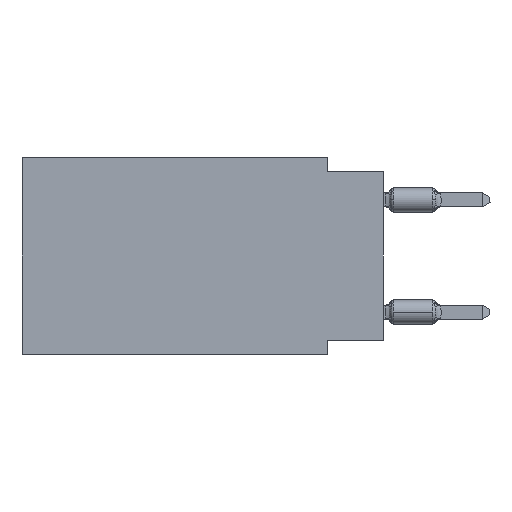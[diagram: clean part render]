
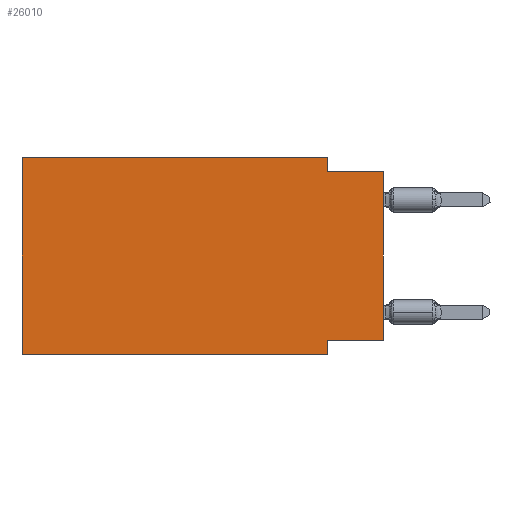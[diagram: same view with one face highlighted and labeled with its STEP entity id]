
A CAD part, left-side view. The second image highlights one B-rep face of the part: STEP entity #26010.
In plain terms, the highlighted planar face has unit normal (-1, 0, 0).
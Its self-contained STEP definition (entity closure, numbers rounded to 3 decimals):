
#1042 = PLANE ( 'NONE',  #23103 ) ;
#2280 = VECTOR ( 'NONE', #2632, 1000. ) ;
#2555 = VERTEX_POINT ( 'NONE', #8932 ) ;
#2632 = DIRECTION ( 'NONE',  ( 0., 1., 0. ) ) ;
#3701 = FACE_OUTER_BOUND ( 'NONE', #25335, .T. ) ;
#4126 = LINE ( 'NONE', #26616, #11478 ) ;
#4437 = LINE ( 'NONE', #19171, #16030 ) ;
#4621 = DIRECTION ( 'NONE',  ( 0., 0., -1. ) ) ;
#4666 = ORIENTED_EDGE ( 'NONE', *, *, #35360, .F. ) ;
#5027 = ORIENTED_EDGE ( 'NONE', *, *, #19436, .F. ) ;
#6119 = CARTESIAN_POINT ( 'NONE',  ( 0., 0., -0.635 ) ) ;
#6375 = DIRECTION ( 'NONE',  ( 0., 0., -1. ) ) ;
#6600 = DIRECTION ( 'NONE',  ( 0., 0., 1. ) ) ;
#7098 = LINE ( 'NONE', #16158, #21920 ) ;
#8932 = CARTESIAN_POINT ( 'NONE',  ( 0., 0., -0.635 ) ) ;
#9439 = VERTEX_POINT ( 'NONE', #15293 ) ;
#10919 = ORIENTED_EDGE ( 'NONE', *, *, #26098, .F. ) ;
#11478 = VECTOR ( 'NONE', #6600, 1000. ) ;
#12414 = DIRECTION ( 'NONE',  ( 1., 0., 0. ) ) ;
#12764 = DIRECTION ( 'NONE',  ( 0., -1., 0. ) ) ;
#13565 = CARTESIAN_POINT ( 'NONE',  ( 0., 2.54, -0.635 ) ) ;
#14224 = VECTOR ( 'NONE', #12764, 1000. ) ;
#14529 = CARTESIAN_POINT ( 'NONE',  ( 0., 2.54, 0. ) ) ;
#14763 = CARTESIAN_POINT ( 'NONE',  ( 0., 0., -8.255 ) ) ;
#15250 = CARTESIAN_POINT ( 'NONE',  ( 0., 16.383, 0. ) ) ;
#15293 = CARTESIAN_POINT ( 'NONE',  ( 0., 16.383, 0. ) ) ;
#15374 = VERTEX_POINT ( 'NONE', #13565 ) ;
#15465 = CARTESIAN_POINT ( 'NONE',  ( 0., 16.383, -8.89 ) ) ;
#15591 = LINE ( 'NONE', #27083, #14224 ) ;
#15969 = CARTESIAN_POINT ( 'NONE',  ( 0., 2.54, -8.89 ) ) ;
#16030 = VECTOR ( 'NONE', #4621, 1000. ) ;
#16158 = CARTESIAN_POINT ( 'NONE',  ( 0., 16.383, 0. ) ) ;
#16815 = CARTESIAN_POINT ( 'NONE',  ( 0., 0., -8.255 ) ) ;
#17197 = LINE ( 'NONE', #16815, #2280 ) ;
#17692 = ORIENTED_EDGE ( 'NONE', *, *, #20731, .F. ) ;
#18241 = ORIENTED_EDGE ( 'NONE', *, *, #19841, .T. ) ;
#18255 = CARTESIAN_POINT ( 'NONE',  ( 0., 16.383, -8.89 ) ) ;
#19171 = CARTESIAN_POINT ( 'NONE',  ( 0., 2.54, -8.89 ) ) ;
#19436 = EDGE_CURVE ( 'NONE', #29420, #21747, #4437, .T. ) ;
#19841 = EDGE_CURVE ( 'NONE', #29462, #21747, #26222, .T. ) ;
#20731 = EDGE_CURVE ( 'NONE', #15374, #2555, #31979, .T. ) ;
#21087 = CARTESIAN_POINT ( 'NONE',  ( 0., 2.54, -8.255 ) ) ;
#21589 = ORIENTED_EDGE ( 'NONE', *, *, #30234, .T. ) ;
#21747 = VERTEX_POINT ( 'NONE', #15969 ) ;
#21920 = VECTOR ( 'NONE', #29944, 1000. ) ;
#23103 = AXIS2_PLACEMENT_3D ( 'NONE', #15250, #12414, #23909 ) ;
#23187 = LINE ( 'NONE', #14529, #33557 ) ;
#23909 = DIRECTION ( 'NONE',  ( 0., 0., -1. ) ) ;
#23943 = DIRECTION ( 'NONE',  ( 0., -1., 0. ) ) ;
#25335 = EDGE_LOOP ( 'NONE', ( #21589, #17692, #28105, #4666, #10919, #18241, #5027, #37055 ) ) ;
#26010 = ADVANCED_FACE ( 'NONE', ( #3701 ), #1042, .F. ) ;
#26098 = EDGE_CURVE ( 'NONE', #29462, #9439, #7098, .T. ) ;
#26222 = LINE ( 'NONE', #15465, #29290 ) ;
#26616 = CARTESIAN_POINT ( 'NONE',  ( 0., 0., 0. ) ) ;
#27083 = CARTESIAN_POINT ( 'NONE',  ( 0., 16.383, 0. ) ) ;
#28105 = ORIENTED_EDGE ( 'NONE', *, *, #33452, .F. ) ;
#29290 = VECTOR ( 'NONE', #23943, 1000. ) ;
#29420 = VERTEX_POINT ( 'NONE', #21087 ) ;
#29462 = VERTEX_POINT ( 'NONE', #18255 ) ;
#29944 = DIRECTION ( 'NONE',  ( 0., 0., 1. ) ) ;
#30234 = EDGE_CURVE ( 'NONE', #34214, #2555, #4126, .T. ) ;
#31501 = CARTESIAN_POINT ( 'NONE',  ( 0., 2.54, 0. ) ) ;
#31723 = EDGE_CURVE ( 'NONE', #34214, #29420, #17197, .T. ) ;
#31790 = DIRECTION ( 'NONE',  ( 0., -1., 0. ) ) ;
#31979 = LINE ( 'NONE', #6119, #33555 ) ;
#33452 = EDGE_CURVE ( 'NONE', #34651, #15374, #23187, .T. ) ;
#33555 = VECTOR ( 'NONE', #31790, 1000. ) ;
#33557 = VECTOR ( 'NONE', #6375, 1000. ) ;
#34214 = VERTEX_POINT ( 'NONE', #14763 ) ;
#34651 = VERTEX_POINT ( 'NONE', #31501 ) ;
#35360 = EDGE_CURVE ( 'NONE', #9439, #34651, #15591, .T. ) ;
#37055 = ORIENTED_EDGE ( 'NONE', *, *, #31723, .F. ) ;
